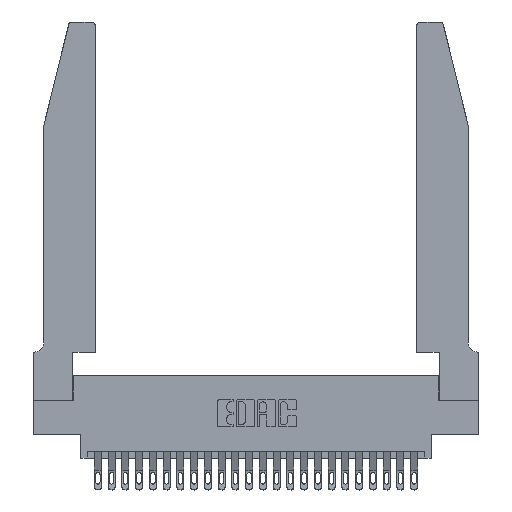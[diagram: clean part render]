
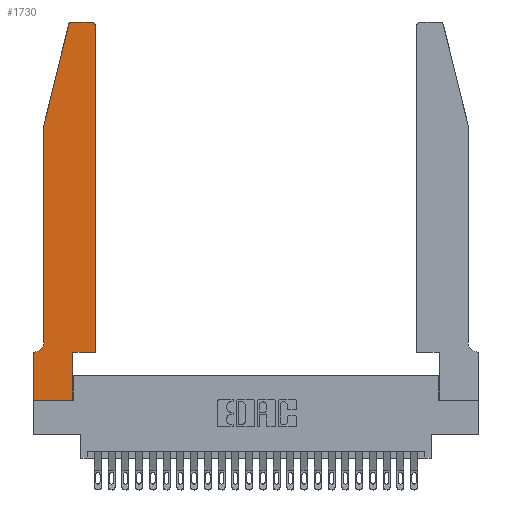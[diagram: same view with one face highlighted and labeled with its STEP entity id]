
A CAD part, top view. The second image highlights one B-rep face of the part: STEP entity #1730.
In plain terms, the highlighted planar face has unit normal (0, 0, 1).
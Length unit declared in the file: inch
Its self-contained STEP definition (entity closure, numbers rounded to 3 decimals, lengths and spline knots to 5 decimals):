
#124 = PLANE ( 'NONE',  #956 ) ;
#289 = DIRECTION ( 'NONE',  ( -0.239, -0.971, 0. ) ) ;
#435 = ORIENTED_EDGE ( 'NONE', *, *, #22891, .T. ) ;
#643 = ORIENTED_EDGE ( 'NONE', *, *, #16793, .T. ) ;
#705 = EDGE_LOOP ( 'NONE', ( #21069, #26334, #7329, #23609, #17088, #19021, #14693, #435, #643, #5218, #8640, #19937 ) ) ;
#956 = AXIS2_PLACEMENT_3D ( 'NONE', #12136, #26057, #14176 ) ;
#1678 = DIRECTION ( 'NONE',  ( 1., 0., 0. ) ) ;
#1730 = ADVANCED_FACE ( 'NONE', ( #4985 ), #124, .T. ) ;
#1946 = VERTEX_POINT ( 'NONE', #10592 ) ;
#1969 = DIRECTION ( 'NONE',  ( 0., 1., 0. ) ) ;
#2029 = CARTESIAN_POINT ( 'NONE',  ( 0.0055, 0.42, 0.37 ) ) ;
#2038 = VERTEX_POINT ( 'NONE', #12941 ) ;
#2091 = CARTESIAN_POINT ( 'NONE',  ( 0.0755, 2., 0.37 ) ) ;
#2180 = CARTESIAN_POINT ( 'NONE',  ( 0., 0., 0.37 ) ) ;
#2578 = EDGE_CURVE ( 'NONE', #16880, #2038, #18949, .T. ) ;
#2621 = EDGE_CURVE ( 'NONE', #23074, #20680, #17714, .T. ) ;
#2817 = AXIS2_PLACEMENT_3D ( 'NONE', #2029, #16513, #4217 ) ;
#3229 = VERTEX_POINT ( 'NONE', #4468 ) ;
#4217 = DIRECTION ( 'NONE',  ( -1., 0., 0. ) ) ;
#4356 = DIRECTION ( 'NONE',  ( 1., 0., 0. ) ) ;
#4468 = CARTESIAN_POINT ( 'NONE',  ( 0.2865, 0., 0.37 ) ) ;
#4738 = CARTESIAN_POINT ( 'NONE',  ( 0., 0., 0.37 ) ) ;
#4814 = CARTESIAN_POINT ( 'NONE',  ( 0.284, 2.75, 0.37 ) ) ;
#4985 = FACE_OUTER_BOUND ( 'NONE', #705, .T. ) ;
#5218 = ORIENTED_EDGE ( 'NONE', *, *, #2621, .T. ) ;
#6839 = VECTOR ( 'NONE', #9614, 39.37008 ) ;
#7131 = EDGE_CURVE ( 'NONE', #20202, #20575, #7541, .T. ) ;
#7204 = EDGE_CURVE ( 'NONE', #18401, #20202, #17083, .T. ) ;
#7329 = ORIENTED_EDGE ( 'NONE', *, *, #7131, .T. ) ;
#7541 = LINE ( 'NONE', #24579, #17715 ) ;
#7752 = EDGE_CURVE ( 'NONE', #20575, #16880, #9740, .T. ) ;
#7797 = CARTESIAN_POINT ( 'NONE',  ( 0.0755, 0.42, 0.37 ) ) ;
#8104 = EDGE_CURVE ( 'NONE', #1946, #18401, #12310, .T. ) ;
#8640 = ORIENTED_EDGE ( 'NONE', *, *, #16192, .T. ) ;
#9004 = CARTESIAN_POINT ( 'NONE',  ( 0.2865, 0.35, 0.37 ) ) ;
#9051 = CARTESIAN_POINT ( 'NONE',  ( 0.284, 2.72, 0.37 ) ) ;
#9088 = CARTESIAN_POINT ( 'NONE',  ( 0., 0.35, 0.37 ) ) ;
#9376 = VERTEX_POINT ( 'NONE', #12168 ) ;
#9438 = CARTESIAN_POINT ( 'NONE',  ( 0.2865, 0.35, 0.37 ) ) ;
#9445 = VECTOR ( 'NONE', #4356, 39.37008 ) ;
#9614 = DIRECTION ( 'NONE',  ( -1., 0., 0. ) ) ;
#9740 = LINE ( 'NONE', #2091, #14562 ) ;
#9825 = EDGE_CURVE ( 'NONE', #16695, #15718, #25048, .T. ) ;
#10291 = AXIS2_PLACEMENT_3D ( 'NONE', #9051, #23107, #11111 ) ;
#10477 = CARTESIAN_POINT ( 'NONE',  ( 0.4505, 0.35, 0.37 ) ) ;
#10592 = CARTESIAN_POINT ( 'NONE',  ( 0.4205, 2.75, 0.37 ) ) ;
#10918 = VECTOR ( 'NONE', #23486, 39.37008 ) ;
#11111 = DIRECTION ( 'NONE',  ( 1., 0., 0. ) ) ;
#11371 = LINE ( 'NONE', #2180, #9445 ) ;
#12136 = CARTESIAN_POINT ( 'NONE',  ( 0., 0.35, 0.37 ) ) ;
#12168 = CARTESIAN_POINT ( 'NONE',  ( 0.4505, 2.72, 0.37 ) ) ;
#12310 = LINE ( 'NONE', #17696, #6839 ) ;
#12538 = DIRECTION ( 'NONE',  ( -1., 0., 0. ) ) ;
#12634 = DIRECTION ( 'NONE',  ( 1., 0., 0. ) ) ;
#12941 = CARTESIAN_POINT ( 'NONE',  ( 0.0055, 0.35, 0.37 ) ) ;
#14137 = LINE ( 'NONE', #18443, #24097 ) ;
#14176 = DIRECTION ( 'NONE',  ( 1., 0., 0. ) ) ;
#14181 = DIRECTION ( 'NONE',  ( 0., 0., 1. ) ) ;
#14562 = VECTOR ( 'NONE', #20556, 39.37008 ) ;
#14693 = ORIENTED_EDGE ( 'NONE', *, *, #9825, .T. ) ;
#15718 = VERTEX_POINT ( 'NONE', #4738 ) ;
#16192 = EDGE_CURVE ( 'NONE', #20680, #9376, #14137, .T. ) ;
#16259 = VECTOR ( 'NONE', #12538, 39.37008 ) ;
#16513 = DIRECTION ( 'NONE',  ( 0., 0., -1. ) ) ;
#16695 = VERTEX_POINT ( 'NONE', #9088 ) ;
#16793 = EDGE_CURVE ( 'NONE', #3229, #23074, #20957, .T. ) ;
#16880 = VERTEX_POINT ( 'NONE', #7797 ) ;
#17082 = VECTOR ( 'NONE', #12634, 39.37008 ) ;
#17083 = CIRCLE ( 'NONE', #10291, 0.03 ) ;
#17088 = ORIENTED_EDGE ( 'NONE', *, *, #2578, .T. ) ;
#17629 = CARTESIAN_POINT ( 'NONE',  ( 0.0755, 2., 0.37 ) ) ;
#17696 = CARTESIAN_POINT ( 'NONE',  ( 0.2605, 2.75, 0.37 ) ) ;
#17714 = LINE ( 'NONE', #10477, #17082 ) ;
#17715 = VECTOR ( 'NONE', #289, 39.37008 ) ;
#18237 = EDGE_CURVE ( 'NONE', #9376, #1946, #20884, .T. ) ;
#18401 = VERTEX_POINT ( 'NONE', #4814 ) ;
#18443 = CARTESIAN_POINT ( 'NONE',  ( 0.4505, 0.35, 0.37 ) ) ;
#18949 = CIRCLE ( 'NONE', #2817, 0.07 ) ;
#19021 = ORIENTED_EDGE ( 'NONE', *, *, #20236, .T. ) ;
#19929 = DIRECTION ( 'NONE',  ( 0., -1., 0. ) ) ;
#19937 = ORIENTED_EDGE ( 'NONE', *, *, #18237, .T. ) ;
#20202 = VERTEX_POINT ( 'NONE', #26277 ) ;
#20236 = EDGE_CURVE ( 'NONE', #2038, #16695, #25562, .T. ) ;
#20556 = DIRECTION ( 'NONE',  ( 0., -1., 0. ) ) ;
#20575 = VERTEX_POINT ( 'NONE', #17629 ) ;
#20680 = VERTEX_POINT ( 'NONE', #23862 ) ;
#20884 = CIRCLE ( 'NONE', #24243, 0.03 ) ;
#20957 = LINE ( 'NONE', #9438, #10918 ) ;
#21069 = ORIENTED_EDGE ( 'NONE', *, *, #8104, .T. ) ;
#22891 = EDGE_CURVE ( 'NONE', #15718, #3229, #11371, .T. ) ;
#23074 = VERTEX_POINT ( 'NONE', #9004 ) ;
#23107 = DIRECTION ( 'NONE',  ( 0., 0., 1. ) ) ;
#23486 = DIRECTION ( 'NONE',  ( 0., 1., 0. ) ) ;
#23609 = ORIENTED_EDGE ( 'NONE', *, *, #7752, .T. ) ;
#23807 = VECTOR ( 'NONE', #19929, 39.37008 ) ;
#23862 = CARTESIAN_POINT ( 'NONE',  ( 0.4505, 0.35, 0.37 ) ) ;
#24097 = VECTOR ( 'NONE', #1969, 39.37008 ) ;
#24243 = AXIS2_PLACEMENT_3D ( 'NONE', #26061, #14181, #1678 ) ;
#24579 = CARTESIAN_POINT ( 'NONE',  ( 0.0755, 2., 0.37 ) ) ;
#25048 = LINE ( 'NONE', #25892, #23807 ) ;
#25562 = LINE ( 'NONE', #26361, #16259 ) ;
#25892 = CARTESIAN_POINT ( 'NONE',  ( 0., 0., 0.37 ) ) ;
#26057 = DIRECTION ( 'NONE',  ( 0., 0., 1. ) ) ;
#26061 = CARTESIAN_POINT ( 'NONE',  ( 0.4205, 2.72, 0.37 ) ) ;
#26277 = CARTESIAN_POINT ( 'NONE',  ( 0.25487, 2.72718, 0.37 ) ) ;
#26334 = ORIENTED_EDGE ( 'NONE', *, *, #7204, .T. ) ;
#26361 = CARTESIAN_POINT ( 'NONE',  ( 0.0755, 0.35, 0.37 ) ) ;
